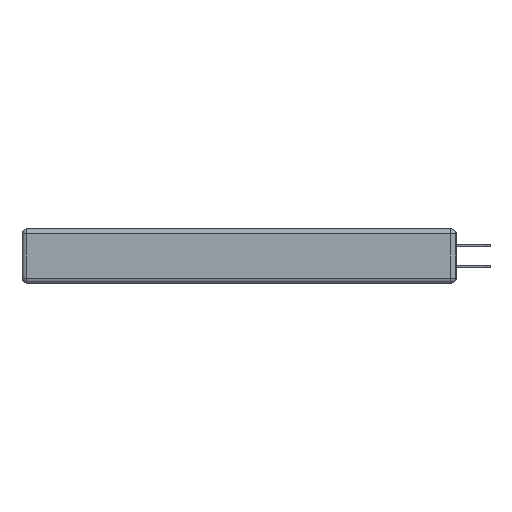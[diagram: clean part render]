
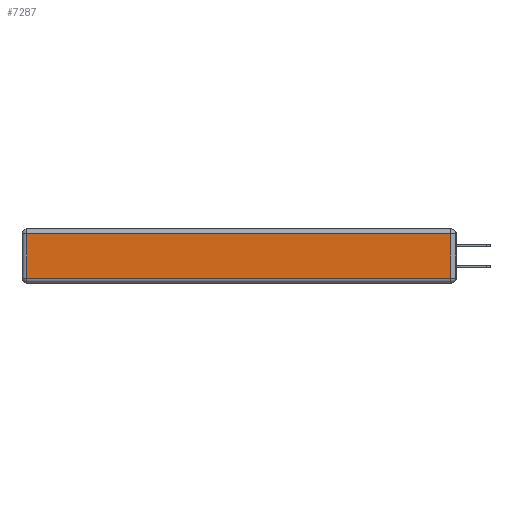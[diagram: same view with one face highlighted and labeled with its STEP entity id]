
A CAD part, left-side view. The second image highlights one B-rep face of the part: STEP entity #7287.
In plain terms, the highlighted planar face has unit normal (-1, 0, 0).
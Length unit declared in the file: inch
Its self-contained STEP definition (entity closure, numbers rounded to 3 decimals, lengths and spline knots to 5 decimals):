
#639 = ORIENTED_EDGE ( 'NONE', *, *, #12209, .T. ) ;
#853 = CARTESIAN_POINT ( 'NONE',  ( 0., 0.03, -0.343 ) ) ;
#920 = DIRECTION ( 'NONE',  ( 0., 0., 1. ) ) ;
#1441 = CARTESIAN_POINT ( 'NONE',  ( 0., 0.03, -0.313 ) ) ;
#2615 = EDGE_LOOP ( 'NONE', ( #3811, #3625, #6463, #639 ) ) ;
#2686 = CARTESIAN_POINT ( 'NONE',  ( 0., 2.72, -0.313 ) ) ;
#2960 = EDGE_CURVE ( 'NONE', #5241, #10614, #5355, .T. ) ;
#3625 = ORIENTED_EDGE ( 'NONE', *, *, #15076, .T. ) ;
#3738 = CARTESIAN_POINT ( 'NONE',  ( 0., 0., -0.313 ) ) ;
#3811 = ORIENTED_EDGE ( 'NONE', *, *, #2960, .T. ) ;
#4174 = VERTEX_POINT ( 'NONE', #4398 ) ;
#4398 = CARTESIAN_POINT ( 'NONE',  ( 0., 2.72, -0.03 ) ) ;
#5134 = DIRECTION ( 'NONE',  ( 0., 1., 0. ) ) ;
#5192 = DIRECTION ( 'NONE',  ( 0., -1., 0. ) ) ;
#5221 = CARTESIAN_POINT ( 'NONE',  ( 0., 0.03, -0.03 ) ) ;
#5241 = VERTEX_POINT ( 'NONE', #2686 ) ;
#5355 = LINE ( 'NONE', #3738, #14890 ) ;
#5691 = CARTESIAN_POINT ( 'NONE',  ( 0., 0., -0.343 ) ) ;
#5810 = LINE ( 'NONE', #8974, #12587 ) ;
#6463 = ORIENTED_EDGE ( 'NONE', *, *, #10684, .T. ) ;
#7287 = ADVANCED_FACE ( 'NONE', ( #13820 ), #11818, .T. ) ;
#8113 = DIRECTION ( 'NONE',  ( -1., 0., 0. ) ) ;
#8511 = VECTOR ( 'NONE', #15067, 39.37008 ) ;
#8920 = DIRECTION ( 'NONE',  ( 0., 0., -1. ) ) ;
#8974 = CARTESIAN_POINT ( 'NONE',  ( 0., 2.72, -0.343 ) ) ;
#9206 = VECTOR ( 'NONE', #5134, 39.37008 ) ;
#10614 = VERTEX_POINT ( 'NONE', #1441 ) ;
#10684 = EDGE_CURVE ( 'NONE', #14787, #4174, #12961, .T. ) ;
#11818 = PLANE ( 'NONE',  #13860 ) ;
#12209 = EDGE_CURVE ( 'NONE', #4174, #5241, #5810, .T. ) ;
#12587 = VECTOR ( 'NONE', #8920, 39.37008 ) ;
#12961 = LINE ( 'NONE', #13602, #9206 ) ;
#13602 = CARTESIAN_POINT ( 'NONE',  ( 0., 2.75, -0.03 ) ) ;
#13820 = FACE_OUTER_BOUND ( 'NONE', #2615, .T. ) ;
#13860 = AXIS2_PLACEMENT_3D ( 'NONE', #5691, #8113, #920 ) ;
#14787 = VERTEX_POINT ( 'NONE', #5221 ) ;
#14883 = LINE ( 'NONE', #853, #8511 ) ;
#14890 = VECTOR ( 'NONE', #5192, 39.37008 ) ;
#15067 = DIRECTION ( 'NONE',  ( 0., 0., 1. ) ) ;
#15076 = EDGE_CURVE ( 'NONE', #10614, #14787, #14883, .T. ) ;
